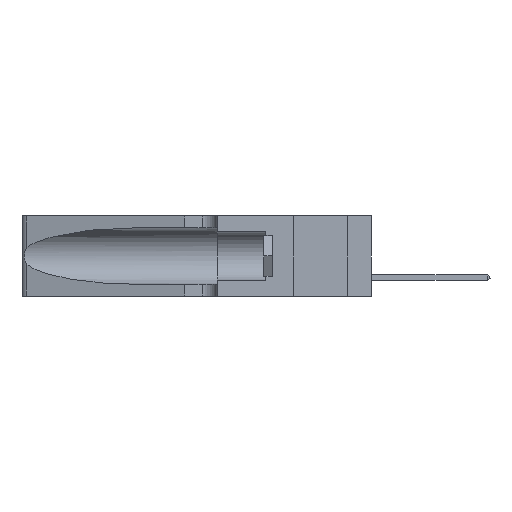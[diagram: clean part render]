
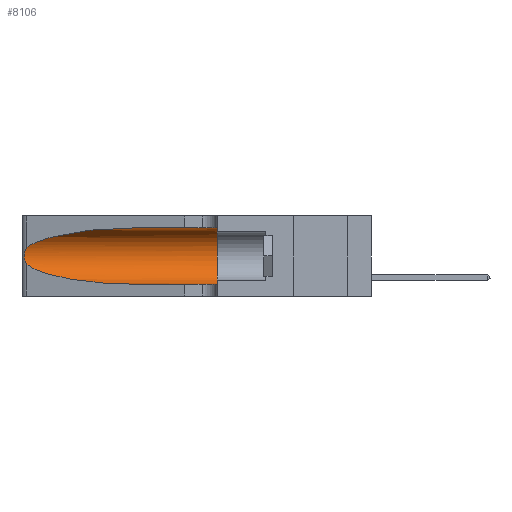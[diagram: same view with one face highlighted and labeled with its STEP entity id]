
A CAD part, left-side view. The second image highlights one B-rep face of the part: STEP entity #8106.
In plain terms, the highlighted cylindrical face has radius 3.308 mm (diameter 6.617 mm), a partial arc.
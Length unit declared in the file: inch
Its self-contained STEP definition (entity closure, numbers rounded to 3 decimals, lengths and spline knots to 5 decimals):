
#712 = AXIS2_PLACEMENT_3D ( 'NONE', #33709, #27090, #33145 ) ;
#1191 = EDGE_CURVE ( 'NONE', #13175, #16015, #36396, .T. ) ;
#1899 = CARTESIAN_POINT ( 'NONE',  ( 0.25789, 1.23486, 0.15765 ) ) ;
#4337 = CARTESIAN_POINT ( 'NONE',  ( 0.25487, 1.22718, 0.14631 ) ) ;
#5030 = CARTESIAN_POINT ( 'NONE',  ( 0.25487, 1.22718, 0.14631 ) ) ;
#6031 = DIRECTION ( 'NONE',  ( 0., 0., -1. ) ) ;
#8106 = ADVANCED_FACE ( 'NONE', ( #8277 ), #36317, .F. ) ;
#8277 = FACE_OUTER_BOUND ( 'NONE', #8962, .T. ) ;
#8962 = EDGE_LOOP ( 'NONE', ( #19379, #33239, #21464, #29358, #25484, #29075 ) ) ;
#9270 = CARTESIAN_POINT ( 'NONE',  ( 0.1305, 0.35, 0.05475 ) ) ;
#10062 = VERTEX_POINT ( 'NONE', #37719 ) ;
#10837 = CARTESIAN_POINT ( 'NONE',  ( 0.25856, 1.23593, 0.16098 ) ) ;
#10968 = CARTESIAN_POINT ( 'NONE',  ( 0.25854, 1.2359, 0.20912 ) ) ;
#11758 = DIRECTION ( 'NONE',  ( 0., -1., 0. ) ) ;
#13175 = VERTEX_POINT ( 'NONE', #33304 ) ;
#13416 = CARTESIAN_POINT ( 'NONE',  ( 0.25487, 1.22718, 0.22369 ) ) ;
#13722 =( BOUNDED_CURVE ( )  B_SPLINE_CURVE ( 3, ( #38712, #32616, #16444, #13416 ),
 .UNSPECIFIED., .F., .F. ) 
 B_SPLINE_CURVE_WITH_KNOTS ( ( 4, 4 ),
 ( 1.5708, 2.84003 ),
 .UNSPECIFIED. ) 
 CURVE ( )  GEOMETRIC_REPRESENTATION_ITEM ( )  RATIONAL_B_SPLINE_CURVE ( ( 1., 0.87, 0.87, 1. ) ) 
 REPRESENTATION_ITEM ( '' )  );
#14060 = EDGE_CURVE ( 'NONE', #25006, #22864, #27963, .T. ) ;
#14244 = CIRCLE ( 'NONE', #712, 0.13025 ) ;
#14375 = DIRECTION ( 'NONE',  ( 0., -1., 0. ) ) ;
#14432 = CARTESIAN_POINT ( 'NONE',  ( 0.26075, 1.23896, 0.178 ) ) ;
#15034 = AXIS2_PLACEMENT_3D ( 'NONE', #21452, #15441, #6031 ) ;
#15068 = CARTESIAN_POINT ( 'NONE',  ( 0.1305, 1.61858, 0.05475 ) ) ;
#15441 = DIRECTION ( 'NONE',  ( 0., -1., 0. ) ) ;
#16015 = VERTEX_POINT ( 'NONE', #22815 ) ;
#16356 = CARTESIAN_POINT ( 'NONE',  ( 0.2373, 1.15595, 0.08982 ) ) ;
#16444 = CARTESIAN_POINT ( 'NONE',  ( 0.2373, 1.15595, 0.28018 ) ) ;
#16486 = CARTESIAN_POINT ( 'NONE',  ( 0.25487, 1.22718, 0.22369 ) ) ;
#18724 = VECTOR ( 'NONE', #14375, 39.37008 ) ;
#19177 = CARTESIAN_POINT ( 'NONE',  ( 0.25487, 1.22718, 0.22369 ) ) ;
#19379 = ORIENTED_EDGE ( 'NONE', *, *, #28359, .T. ) ;
#19626 = CARTESIAN_POINT ( 'NONE',  ( 0.26018, 1.23835, 0.19895 ) ) ;
#19766 = B_SPLINE_CURVE_WITH_KNOTS ( 'NONE', 3,
 ( #16486, #38463, #25902, #33203, #10968, #19626, #23451, #14432, #39560, #10837, #1899, #39289, #23870, #5030 ),
 .UNSPECIFIED., .F., .F.,
 ( 4, 2, 2, 2, 2, 2, 4 ),
 ( 0., 0.00027, 0.00053, 0.00107, 0.0016, 0.00187, 0.00214 ),
 .UNSPECIFIED. ) ;
#21452 = CARTESIAN_POINT ( 'NONE',  ( 0.1305, 1.61858, 0.185 ) ) ;
#21464 = ORIENTED_EDGE ( 'NONE', *, *, #35882, .T. ) ;
#22815 = CARTESIAN_POINT ( 'NONE',  ( 0.1305, 0.35, 0.31525 ) ) ;
#22864 = VERTEX_POINT ( 'NONE', #9270 ) ;
#23451 = CARTESIAN_POINT ( 'NONE',  ( 0.26075, 1.23896, 0.19203 ) ) ;
#23870 = CARTESIAN_POINT ( 'NONE',  ( 0.25555, 1.22993, 0.14849 ) ) ;
#25006 = VERTEX_POINT ( 'NONE', #28449 ) ;
#25484 = ORIENTED_EDGE ( 'NONE', *, *, #33027, .F. ) ;
#25902 = CARTESIAN_POINT ( 'NONE',  ( 0.25639, 1.23184, 0.21858 ) ) ;
#25957 = VECTOR ( 'NONE', #11758, 39.37008 ) ;
#26161 = CARTESIAN_POINT ( 'NONE',  ( 0.1305, 0.72297, 0.05475 ) ) ;
#27090 = DIRECTION ( 'NONE',  ( 0., 1., 0. ) ) ;
#27963 = LINE ( 'NONE', #15068, #25957 ) ;
#28359 = EDGE_CURVE ( 'NONE', #13175, #30938, #13722, .T. ) ;
#28449 = CARTESIAN_POINT ( 'NONE',  ( 0.1305, 0.72297, 0.05475 ) ) ;
#29075 = ORIENTED_EDGE ( 'NONE', *, *, #1191, .F. ) ;
#29358 = ORIENTED_EDGE ( 'NONE', *, *, #14060, .T. ) ;
#30938 = VERTEX_POINT ( 'NONE', #19177 ) ;
#31335 =( BOUNDED_CURVE ( )  B_SPLINE_CURVE ( 3, ( #4337, #16356, #35417, #26161 ),
 .UNSPECIFIED., .F., .F. ) 
 B_SPLINE_CURVE_WITH_KNOTS ( ( 4, 4 ),
 ( 3.44316, 4.71239 ),
 .UNSPECIFIED. ) 
 CURVE ( )  GEOMETRIC_REPRESENTATION_ITEM ( )  RATIONAL_B_SPLINE_CURVE ( ( 1., 0.87, 0.87, 1. ) ) 
 REPRESENTATION_ITEM ( '' )  );
#32616 = CARTESIAN_POINT ( 'NONE',  ( 0.18966, 0.96281, 0.31525 ) ) ;
#33027 = EDGE_CURVE ( 'NONE', #16015, #22864, #14244, .T. ) ;
#33145 = DIRECTION ( 'NONE',  ( 0., 0., 1. ) ) ;
#33203 = CARTESIAN_POINT ( 'NONE',  ( 0.25787, 1.23484, 0.2124 ) ) ;
#33239 = ORIENTED_EDGE ( 'NONE', *, *, #37049, .T. ) ;
#33304 = CARTESIAN_POINT ( 'NONE',  ( 0.1305, 0.72297, 0.31525 ) ) ;
#33709 = CARTESIAN_POINT ( 'NONE',  ( 0.1305, 0.35, 0.185 ) ) ;
#35417 = CARTESIAN_POINT ( 'NONE',  ( 0.18966, 0.96281, 0.05475 ) ) ;
#35882 = EDGE_CURVE ( 'NONE', #10062, #25006, #31335, .T. ) ;
#36317 = CYLINDRICAL_SURFACE ( 'NONE', #15034, 0.13025 ) ;
#36331 = CARTESIAN_POINT ( 'NONE',  ( 0.1305, 1.61858, 0.31525 ) ) ;
#36396 = LINE ( 'NONE', #36331, #18724 ) ;
#37049 = EDGE_CURVE ( 'NONE', #30938, #10062, #19766, .T. ) ;
#37719 = CARTESIAN_POINT ( 'NONE',  ( 0.25487, 1.22718, 0.14631 ) ) ;
#38463 = CARTESIAN_POINT ( 'NONE',  ( 0.25555, 1.22994, 0.2215 ) ) ;
#38712 = CARTESIAN_POINT ( 'NONE',  ( 0.1305, 0.72297, 0.31525 ) ) ;
#39289 = CARTESIAN_POINT ( 'NONE',  ( 0.25639, 1.23186, 0.15144 ) ) ;
#39560 = CARTESIAN_POINT ( 'NONE',  ( 0.26017, 1.23833, 0.17102 ) ) ;
